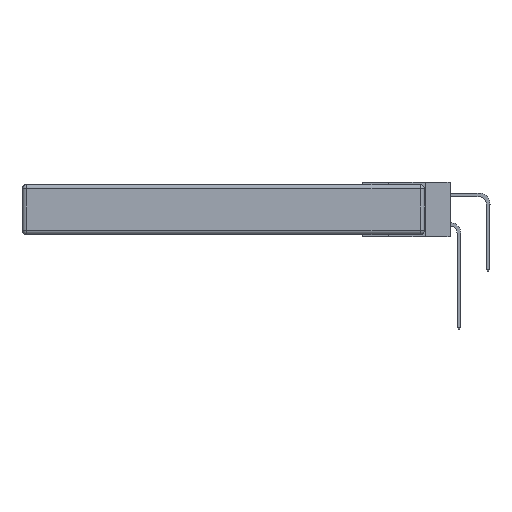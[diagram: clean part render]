
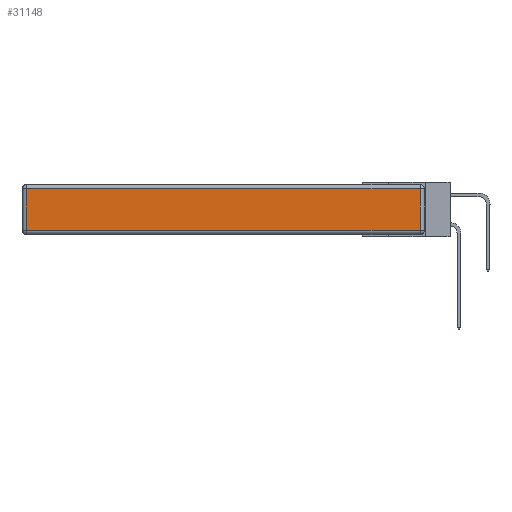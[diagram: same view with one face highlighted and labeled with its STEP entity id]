
A CAD part, left-side view. The second image highlights one B-rep face of the part: STEP entity #31148.
In plain terms, the highlighted planar face has unit normal (-1, 0, 0).
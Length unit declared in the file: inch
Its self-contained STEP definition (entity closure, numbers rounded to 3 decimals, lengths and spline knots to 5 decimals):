
#119 = CARTESIAN_POINT ( 'NONE',  ( 0., 0.03, -0.343 ) ) ;
#1838 = CARTESIAN_POINT ( 'NONE',  ( 0., 0., -0.343 ) ) ;
#4236 = ORIENTED_EDGE ( 'NONE', *, *, #19735, .T. ) ;
#4673 = VERTEX_POINT ( 'NONE', #27678 ) ;
#7067 = CARTESIAN_POINT ( 'NONE',  ( 0., 0.03, -0.313 ) ) ;
#7551 = CARTESIAN_POINT ( 'NONE',  ( 0., 0.03, -0.03 ) ) ;
#9341 = VERTEX_POINT ( 'NONE', #7067 ) ;
#10282 = CARTESIAN_POINT ( 'NONE',  ( 0., 2.75, -0.03 ) ) ;
#10346 = DIRECTION ( 'NONE',  ( 0., 0., 1. ) ) ;
#10448 = ORIENTED_EDGE ( 'NONE', *, *, #13180, .T. ) ;
#13034 = PLANE ( 'NONE',  #13757 ) ;
#13180 = EDGE_CURVE ( 'NONE', #32891, #4673, #24190, .T. ) ;
#13757 = AXIS2_PLACEMENT_3D ( 'NONE', #1838, #15906, #10346 ) ;
#15906 = DIRECTION ( 'NONE',  ( -1., 0., 0. ) ) ;
#15957 = DIRECTION ( 'NONE',  ( 0., 0., -1. ) ) ;
#18525 = CARTESIAN_POINT ( 'NONE',  ( 0., 2.72, -0.313 ) ) ;
#19489 = VECTOR ( 'NONE', #23364, 39.37008 ) ;
#19735 = EDGE_CURVE ( 'NONE', #4673, #25176, #35409, .T. ) ;
#21282 = LINE ( 'NONE', #119, #19489 ) ;
#21869 = VECTOR ( 'NONE', #15957, 39.37008 ) ;
#23364 = DIRECTION ( 'NONE',  ( 0., 0., 1. ) ) ;
#24190 = LINE ( 'NONE', #10282, #36806 ) ;
#25176 = VERTEX_POINT ( 'NONE', #18525 ) ;
#25423 = EDGE_CURVE ( 'NONE', #9341, #32891, #21282, .T. ) ;
#25540 = EDGE_CURVE ( 'NONE', #25176, #9341, #27111, .T. ) ;
#26254 = VECTOR ( 'NONE', #32183, 39.37008 ) ;
#27111 = LINE ( 'NONE', #29263, #26254 ) ;
#27678 = CARTESIAN_POINT ( 'NONE',  ( 0., 2.72, -0.03 ) ) ;
#29263 = CARTESIAN_POINT ( 'NONE',  ( 0., 0., -0.313 ) ) ;
#29550 = ORIENTED_EDGE ( 'NONE', *, *, #25423, .T. ) ;
#30174 = CARTESIAN_POINT ( 'NONE',  ( 0., 2.72, -0.343 ) ) ;
#30403 = DIRECTION ( 'NONE',  ( 0., 1., 0. ) ) ;
#31148 = ADVANCED_FACE ( 'NONE', ( #32564 ), #13034, .T. ) ;
#32183 = DIRECTION ( 'NONE',  ( 0., -1., 0. ) ) ;
#32564 = FACE_OUTER_BOUND ( 'NONE', #35397, .T. ) ;
#32658 = ORIENTED_EDGE ( 'NONE', *, *, #25540, .T. ) ;
#32891 = VERTEX_POINT ( 'NONE', #7551 ) ;
#35397 = EDGE_LOOP ( 'NONE', ( #32658, #29550, #10448, #4236 ) ) ;
#35409 = LINE ( 'NONE', #30174, #21869 ) ;
#36806 = VECTOR ( 'NONE', #30403, 39.37008 ) ;
